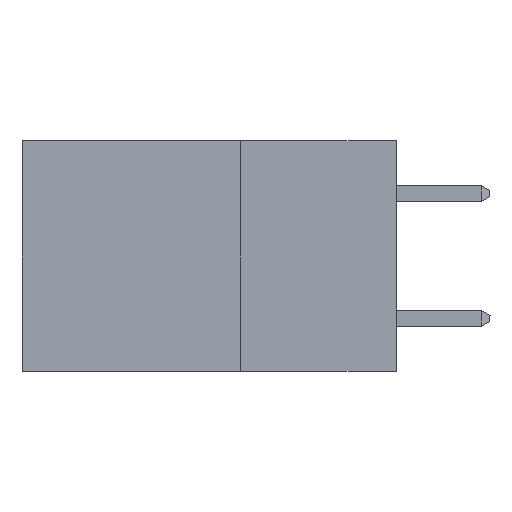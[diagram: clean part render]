
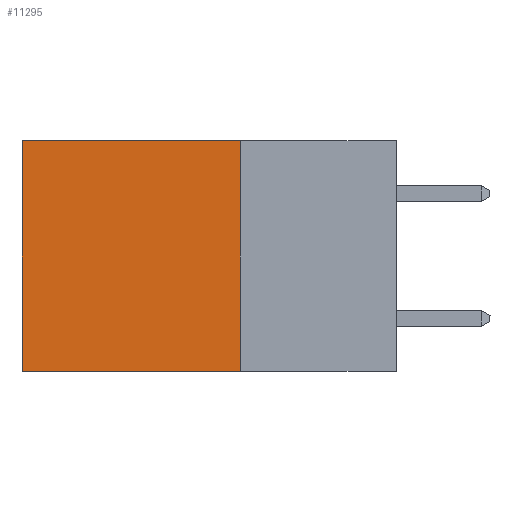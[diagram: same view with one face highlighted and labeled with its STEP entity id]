
A CAD part, left-side view. The second image highlights one B-rep face of the part: STEP entity #11295.
In plain terms, the highlighted planar face has unit normal (-1, 0, 0).
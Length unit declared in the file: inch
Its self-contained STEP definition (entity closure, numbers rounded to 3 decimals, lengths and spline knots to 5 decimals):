
#157 = CARTESIAN_POINT ( 'NONE',  ( 0.2615, 0.6, 0. ) ) ;
#1146 = DIRECTION ( 'NONE',  ( 1., 0., 0. ) ) ;
#1634 = FACE_OUTER_BOUND ( 'NONE', #3406, .T. ) ;
#2410 = LINE ( 'NONE', #12982, #5908 ) ;
#2931 = LINE ( 'NONE', #14104, #9472 ) ;
#3406 = EDGE_LOOP ( 'NONE', ( #11779, #16718, #9467, #9669 ) ) ;
#3798 = VERTEX_POINT ( 'NONE', #7554 ) ;
#4536 = CARTESIAN_POINT ( 'NONE',  ( 0.2615, 0.25, -0.37 ) ) ;
#5846 = DIRECTION ( 'NONE',  ( 0., 0., -1. ) ) ;
#5908 = VECTOR ( 'NONE', #15457, 39.37008 ) ;
#5940 = AXIS2_PLACEMENT_3D ( 'NONE', #9037, #1146, #10373 ) ;
#6842 = VERTEX_POINT ( 'NONE', #15726 ) ;
#7360 = VERTEX_POINT ( 'NONE', #8025 ) ;
#7554 = CARTESIAN_POINT ( 'NONE',  ( 0.2615, 0.6, -0.37 ) ) ;
#7695 = DIRECTION ( 'NONE',  ( 0., 1., 0. ) ) ;
#8025 = CARTESIAN_POINT ( 'NONE',  ( 0.2615, 0.25, -0.37 ) ) ;
#9037 = CARTESIAN_POINT ( 'NONE',  ( 0.2615, 0.25, -0.37 ) ) ;
#9467 = ORIENTED_EDGE ( 'NONE', *, *, #15008, .F. ) ;
#9472 = VECTOR ( 'NONE', #13917, 39.37008 ) ;
#9669 = ORIENTED_EDGE ( 'NONE', *, *, #13310, .T. ) ;
#9744 = LINE ( 'NONE', #4536, #16075 ) ;
#9800 = VERTEX_POINT ( 'NONE', #157 ) ;
#9853 = EDGE_CURVE ( 'NONE', #9800, #3798, #2931, .T. ) ;
#10373 = DIRECTION ( 'NONE',  ( 0., 0., -1. ) ) ;
#11295 = ADVANCED_FACE ( 'NONE', ( #1634 ), #16635, .F. ) ;
#11779 = ORIENTED_EDGE ( 'NONE', *, *, #9853, .T. ) ;
#12010 = EDGE_CURVE ( 'NONE', #7360, #3798, #15570, .T. ) ;
#12982 = CARTESIAN_POINT ( 'NONE',  ( 0.2615, 0.25, 0. ) ) ;
#13310 = EDGE_CURVE ( 'NONE', #6842, #9800, #2410, .T. ) ;
#13917 = DIRECTION ( 'NONE',  ( 0., 0., -1. ) ) ;
#14104 = CARTESIAN_POINT ( 'NONE',  ( 0.2615, 0.6, -0.37 ) ) ;
#14176 = CARTESIAN_POINT ( 'NONE',  ( 0.2615, 0.25, -0.37 ) ) ;
#14817 = VECTOR ( 'NONE', #7695, 39.37008 ) ;
#15008 = EDGE_CURVE ( 'NONE', #6842, #7360, #9744, .T. ) ;
#15457 = DIRECTION ( 'NONE',  ( 0., 1., 0. ) ) ;
#15570 = LINE ( 'NONE', #14176, #14817 ) ;
#15726 = CARTESIAN_POINT ( 'NONE',  ( 0.2615, 0.25, 0. ) ) ;
#16075 = VECTOR ( 'NONE', #5846, 39.37008 ) ;
#16635 = PLANE ( 'NONE',  #5940 ) ;
#16718 = ORIENTED_EDGE ( 'NONE', *, *, #12010, .F. ) ;
